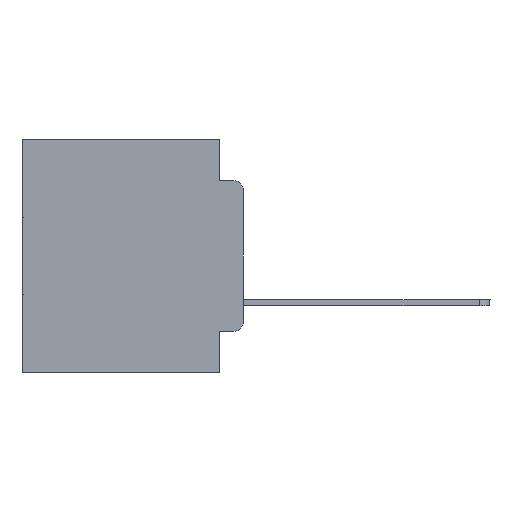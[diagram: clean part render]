
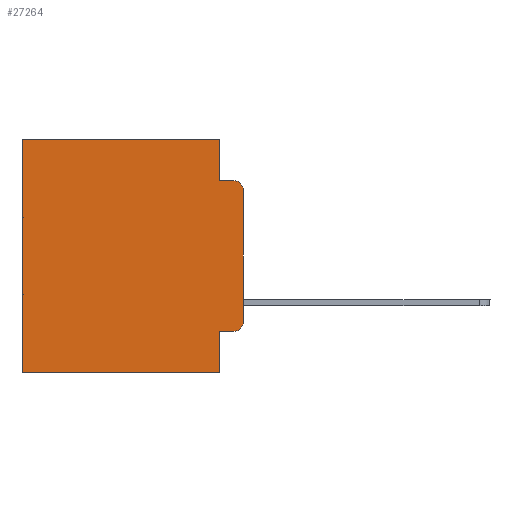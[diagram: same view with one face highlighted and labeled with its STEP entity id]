
A CAD part, left-side view. The second image highlights one B-rep face of the part: STEP entity #27264.
In plain terms, the highlighted planar face has unit normal (-1, 0, 0).
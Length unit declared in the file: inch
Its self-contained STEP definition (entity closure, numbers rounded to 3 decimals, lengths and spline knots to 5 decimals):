
#477 = ORIENTED_EDGE ( 'NONE', *, *, #4183, .F. ) ;
#733 = FACE_OUTER_BOUND ( 'NONE', #28237, .T. ) ;
#1280 = CARTESIAN_POINT ( 'NONE',  ( 0.298, 0.051, -0.0885 ) ) ;
#1461 = AXIS2_PLACEMENT_3D ( 'NONE', #12682, #3028, #27795 ) ;
#1730 = CARTESIAN_POINT ( 'NONE',  ( 0.298, 0.051, 0. ) ) ;
#1784 = EDGE_CURVE ( 'NONE', #16011, #17760, #22533, .T. ) ;
#1984 = DIRECTION ( 'NONE',  ( 0., 0., -1. ) ) ;
#2181 = VERTEX_POINT ( 'NONE', #9652 ) ;
#2671 = VECTOR ( 'NONE', #1984, 39.37008 ) ;
#3028 = DIRECTION ( 'NONE',  ( 1., 0., 0. ) ) ;
#3112 = CARTESIAN_POINT ( 'NONE',  ( 0.298, 0., 0. ) ) ;
#3423 = DIRECTION ( 'NONE',  ( 0., -1., 0. ) ) ;
#3824 = LINE ( 'NONE', #9309, #2671 ) ;
#4006 = VERTEX_POINT ( 'NONE', #1280 ) ;
#4103 = DIRECTION ( 'NONE',  ( 0., 0., -1. ) ) ;
#4183 = EDGE_CURVE ( 'NONE', #2181, #31427, #12392, .T. ) ;
#4623 = VERTEX_POINT ( 'NONE', #22073 ) ;
#4859 = CARTESIAN_POINT ( 'NONE',  ( 0.298, 0.02, -0.1085 ) ) ;
#6514 = DIRECTION ( 'NONE',  ( 0., 0., -1. ) ) ;
#7483 = DIRECTION ( 'NONE',  ( 0., 1., 0. ) ) ;
#7886 = LINE ( 'NONE', #23974, #9482 ) ;
#9132 = LINE ( 'NONE', #21993, #28874 ) ;
#9309 = CARTESIAN_POINT ( 'NONE',  ( 0.298, 0.051, 0. ) ) ;
#9482 = VECTOR ( 'NONE', #6514, 39.37008 ) ;
#9652 = CARTESIAN_POINT ( 'NONE',  ( 0.298, 0.051, -0.5 ) ) ;
#9825 = VERTEX_POINT ( 'NONE', #20142 ) ;
#10048 = AXIS2_PLACEMENT_3D ( 'NONE', #4859, #26853, #29652 ) ;
#10166 = ORIENTED_EDGE ( 'NONE', *, *, #21213, .F. ) ;
#10181 = ORIENTED_EDGE ( 'NONE', *, *, #10885, .F. ) ;
#10286 = ORIENTED_EDGE ( 'NONE', *, *, #28068, .T. ) ;
#10497 = PLANE ( 'NONE',  #1461 ) ;
#10885 = EDGE_CURVE ( 'NONE', #11151, #4006, #9132, .T. ) ;
#10934 = EDGE_CURVE ( 'NONE', #16011, #4623, #21517, .T. ) ;
#11151 = VERTEX_POINT ( 'NONE', #1730 ) ;
#11273 = DIRECTION ( 'NONE',  ( 0., -1., 0. ) ) ;
#11454 = DIRECTION ( 'NONE',  ( 0., 0., -1. ) ) ;
#11541 = EDGE_CURVE ( 'NONE', #9825, #31427, #7886, .T. ) ;
#11878 = EDGE_CURVE ( 'NONE', #4006, #17760, #22229, .T. ) ;
#12392 = LINE ( 'NONE', #19936, #15467 ) ;
#12532 = VECTOR ( 'NONE', #3423, 39.37008 ) ;
#12638 = ORIENTED_EDGE ( 'NONE', *, *, #1784, .T. ) ;
#12682 = CARTESIAN_POINT ( 'NONE',  ( 0.298, 0., 0. ) ) ;
#12910 = CARTESIAN_POINT ( 'NONE',  ( 0.298, 0.02, -0.0885 ) ) ;
#13307 = DIRECTION ( 'NONE',  ( 0., 1., 0. ) ) ;
#13666 = ORIENTED_EDGE ( 'NONE', *, *, #11878, .F. ) ;
#14430 = ORIENTED_EDGE ( 'NONE', *, *, #17171, .T. ) ;
#14887 = LINE ( 'NONE', #26107, #30765 ) ;
#15379 = AXIS2_PLACEMENT_3D ( 'NONE', #24253, #21510, #4103 ) ;
#15467 = VECTOR ( 'NONE', #7483, 39.37008 ) ;
#16011 = VERTEX_POINT ( 'NONE', #20077 ) ;
#16045 = VERTEX_POINT ( 'NONE', #29060 ) ;
#17171 = EDGE_CURVE ( 'NONE', #16045, #4623, #31948, .T. ) ;
#17760 = VERTEX_POINT ( 'NONE', #12910 ) ;
#17933 = CARTESIAN_POINT ( 'NONE',  ( 0.298, 0.473, -0.5 ) ) ;
#19936 = CARTESIAN_POINT ( 'NONE',  ( 0.298, 0., -0.5 ) ) ;
#20077 = CARTESIAN_POINT ( 'NONE',  ( 0.298, 0., -0.1085 ) ) ;
#20142 = CARTESIAN_POINT ( 'NONE',  ( 0.298, 0.473, 0. ) ) ;
#21208 = VECTOR ( 'NONE', #13307, 39.37008 ) ;
#21213 = EDGE_CURVE ( 'NONE', #31586, #2181, #3824, .T. ) ;
#21510 = DIRECTION ( 'NONE',  ( -1., 0., 0. ) ) ;
#21517 = LINE ( 'NONE', #28507, #22280 ) ;
#21993 = CARTESIAN_POINT ( 'NONE',  ( 0.298, 0.051, 0. ) ) ;
#22073 = CARTESIAN_POINT ( 'NONE',  ( 0.298, 0., -0.3915 ) ) ;
#22229 = LINE ( 'NONE', #28308, #12532 ) ;
#22280 = VECTOR ( 'NONE', #11454, 39.37008 ) ;
#22533 = CIRCLE ( 'NONE', #10048, 0.02 ) ;
#23340 = EDGE_CURVE ( 'NONE', #31586, #16045, #14887, .T. ) ;
#23974 = CARTESIAN_POINT ( 'NONE',  ( 0.298, 0.473, 0. ) ) ;
#24132 = CARTESIAN_POINT ( 'NONE',  ( 0.298, 0.051, -0.4115 ) ) ;
#24253 = CARTESIAN_POINT ( 'NONE',  ( 0.298, 0.02, -0.3915 ) ) ;
#26107 = CARTESIAN_POINT ( 'NONE',  ( 0.298, 0.051, -0.4115 ) ) ;
#26757 = ORIENTED_EDGE ( 'NONE', *, *, #11541, .T. ) ;
#26853 = DIRECTION ( 'NONE',  ( -1., 0., 0. ) ) ;
#27264 = ADVANCED_FACE ( 'NONE', ( #733 ), #10497, .F. ) ;
#27763 = LINE ( 'NONE', #3112, #21208 ) ;
#27795 = DIRECTION ( 'NONE',  ( 0., 0., -1. ) ) ;
#27997 = ORIENTED_EDGE ( 'NONE', *, *, #23340, .T. ) ;
#28068 = EDGE_CURVE ( 'NONE', #11151, #9825, #27763, .T. ) ;
#28237 = EDGE_LOOP ( 'NONE', ( #30475, #12638, #13666, #10181, #10286, #26757, #477, #10166, #27997, #14430 ) ) ;
#28308 = CARTESIAN_POINT ( 'NONE',  ( 0.298, 0.051, -0.0885 ) ) ;
#28507 = CARTESIAN_POINT ( 'NONE',  ( 0.298, 0., 0. ) ) ;
#28874 = VECTOR ( 'NONE', #29254, 39.37008 ) ;
#29060 = CARTESIAN_POINT ( 'NONE',  ( 0.298, 0.02, -0.4115 ) ) ;
#29254 = DIRECTION ( 'NONE',  ( 0., 0., -1. ) ) ;
#29652 = DIRECTION ( 'NONE',  ( 0., 0., -1. ) ) ;
#30475 = ORIENTED_EDGE ( 'NONE', *, *, #10934, .F. ) ;
#30765 = VECTOR ( 'NONE', #11273, 39.37008 ) ;
#31427 = VERTEX_POINT ( 'NONE', #17933 ) ;
#31586 = VERTEX_POINT ( 'NONE', #24132 ) ;
#31948 = CIRCLE ( 'NONE', #15379, 0.02 ) ;
